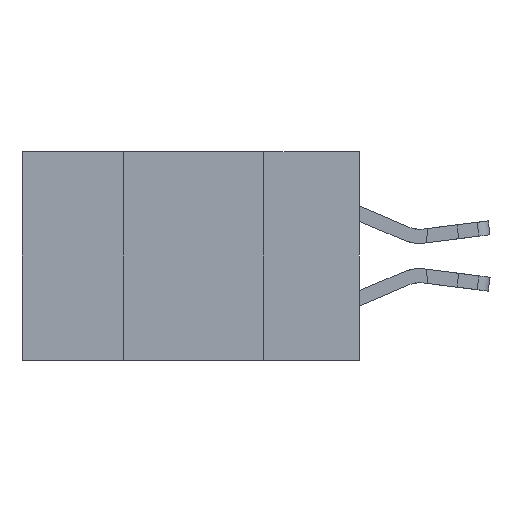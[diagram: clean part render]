
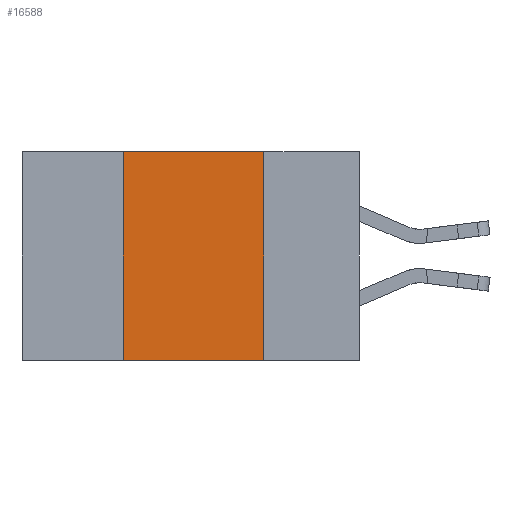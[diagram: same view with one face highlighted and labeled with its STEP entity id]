
A CAD part, left-side view. The second image highlights one B-rep face of the part: STEP entity #16588.
In plain terms, the highlighted planar face has unit normal (-1, 0, 0).
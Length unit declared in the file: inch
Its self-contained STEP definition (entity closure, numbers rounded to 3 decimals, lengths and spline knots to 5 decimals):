
#129 = CARTESIAN_POINT ( 'NONE',  ( 0., 0.6, 0. ) ) ;
#965 = EDGE_LOOP ( 'NONE', ( #13419, #3387, #10321, #2148 ) ) ;
#1059 = CARTESIAN_POINT ( 'NONE',  ( 0., 0.42, 0. ) ) ;
#2148 = ORIENTED_EDGE ( 'NONE', *, *, #12814, .T. ) ;
#2583 = AXIS2_PLACEMENT_3D ( 'NONE', #129, #10906, #10768 ) ;
#3387 = ORIENTED_EDGE ( 'NONE', *, *, #4137, .F. ) ;
#3756 = LINE ( 'NONE', #14192, #12106 ) ;
#4137 = EDGE_CURVE ( 'NONE', #10965, #14428, #17831, .T. ) ;
#4320 = CARTESIAN_POINT ( 'NONE',  ( 0., 0.17, -0.37 ) ) ;
#6009 = EDGE_CURVE ( 'NONE', #14428, #15162, #11575, .T. ) ;
#6096 = CARTESIAN_POINT ( 'NONE',  ( 0., 0.42, 0. ) ) ;
#7001 = CARTESIAN_POINT ( 'NONE',  ( 0., 0.17, 0. ) ) ;
#8203 = VERTEX_POINT ( 'NONE', #16671 ) ;
#8999 = DIRECTION ( 'NONE',  ( 0., 0., -1. ) ) ;
#9373 = DIRECTION ( 'NONE',  ( 0., -1., 0. ) ) ;
#9417 = PLANE ( 'NONE',  #2583 ) ;
#10321 = ORIENTED_EDGE ( 'NONE', *, *, #13225, .F. ) ;
#10440 = VECTOR ( 'NONE', #19529, 39.37008 ) ;
#10768 = DIRECTION ( 'NONE',  ( 0., 0., -1. ) ) ;
#10906 = DIRECTION ( 'NONE',  ( 1., 0., 0. ) ) ;
#10965 = VERTEX_POINT ( 'NONE', #1059 ) ;
#11575 = LINE ( 'NONE', #16356, #16523 ) ;
#12106 = VECTOR ( 'NONE', #9373, 39.37008 ) ;
#12114 = CARTESIAN_POINT ( 'NONE',  ( 0., 0.6, 0. ) ) ;
#12555 = LINE ( 'NONE', #6096, #10440 ) ;
#12814 = EDGE_CURVE ( 'NONE', #8203, #15162, #3756, .T. ) ;
#13225 = EDGE_CURVE ( 'NONE', #8203, #10965, #12555, .T. ) ;
#13419 = ORIENTED_EDGE ( 'NONE', *, *, #6009, .F. ) ;
#13632 = DIRECTION ( 'NONE',  ( 0., -1., 0. ) ) ;
#13810 = VECTOR ( 'NONE', #13632, 39.37008 ) ;
#14192 = CARTESIAN_POINT ( 'NONE',  ( 0., 0.6, -0.37 ) ) ;
#14428 = VERTEX_POINT ( 'NONE', #7001 ) ;
#15162 = VERTEX_POINT ( 'NONE', #4320 ) ;
#16356 = CARTESIAN_POINT ( 'NONE',  ( 0., 0.17, 0. ) ) ;
#16523 = VECTOR ( 'NONE', #8999, 39.37008 ) ;
#16588 = ADVANCED_FACE ( 'NONE', ( #17283 ), #9417, .F. ) ;
#16671 = CARTESIAN_POINT ( 'NONE',  ( 0., 0.42, -0.37 ) ) ;
#17283 = FACE_OUTER_BOUND ( 'NONE', #965, .T. ) ;
#17831 = LINE ( 'NONE', #12114, #13810 ) ;
#19529 = DIRECTION ( 'NONE',  ( 0., 0., 1. ) ) ;
